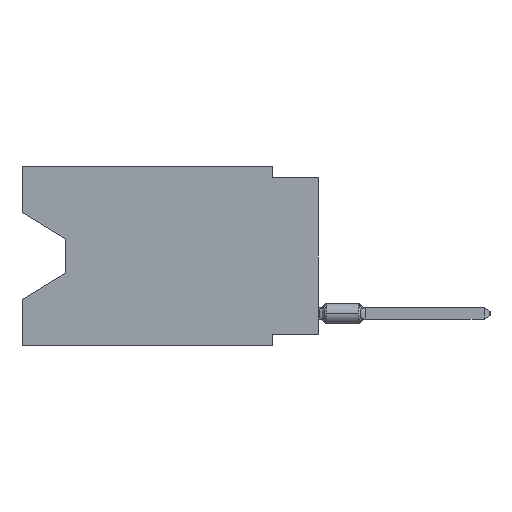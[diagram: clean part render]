
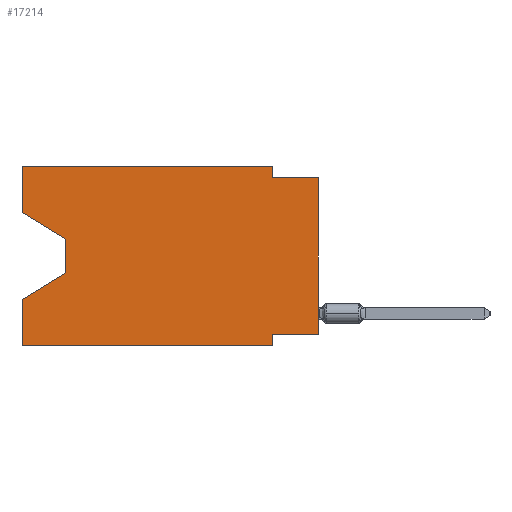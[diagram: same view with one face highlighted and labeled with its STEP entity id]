
A CAD part, left-side view. The second image highlights one B-rep face of the part: STEP entity #17214.
In plain terms, the highlighted planar face has unit normal (-1, 0, 0).
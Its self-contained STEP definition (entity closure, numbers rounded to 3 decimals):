
#974 = LINE ( 'NONE', #6072, #51838 ) ;
#1066 = VERTEX_POINT ( 'NONE', #37199 ) ;
#1993 = DIRECTION ( 'NONE',  ( 0., 0., -1. ) ) ;
#2234 = CARTESIAN_POINT ( 'NONE',  ( 0., 0., -0.635 ) ) ;
#3231 = ORIENTED_EDGE ( 'NONE', *, *, #65630, .T. ) ;
#3848 = CARTESIAN_POINT ( 'NONE',  ( 0., 16.383, -2.546 ) ) ;
#4246 = CARTESIAN_POINT ( 'NONE',  ( 0., 16.383, 0. ) ) ;
#5238 = DIRECTION ( 'NONE',  ( 0., 1., 0. ) ) ;
#5578 = LINE ( 'NONE', #27702, #69295 ) ;
#5609 = DIRECTION ( 'NONE',  ( 0., -0.855, -0.519 ) ) ;
#5758 = CARTESIAN_POINT ( 'NONE',  ( 0., 0., -0.635 ) ) ;
#5978 = EDGE_CURVE ( 'NONE', #13205, #69093, #974, .T. ) ;
#6072 = CARTESIAN_POINT ( 'NONE',  ( 0., 13.97, -5.893 ) ) ;
#9314 = EDGE_CURVE ( 'NONE', #17321, #13205, #5578, .T. ) ;
#12777 = VECTOR ( 'NONE', #44571, 1000. ) ;
#13205 = VERTEX_POINT ( 'NONE', #16826 ) ;
#14056 = VERTEX_POINT ( 'NONE', #45647 ) ;
#14090 = CARTESIAN_POINT ( 'NONE',  ( 0., 16.383, -7.36 ) ) ;
#15935 = PLANE ( 'NONE',  #58836 ) ;
#16826 = CARTESIAN_POINT ( 'NONE',  ( 0., 13.97, -5.893 ) ) ;
#17214 = ADVANCED_FACE ( 'NONE', ( #64526 ), #15935, .F. ) ;
#17321 = VERTEX_POINT ( 'NONE', #65959 ) ;
#18613 = EDGE_CURVE ( 'NONE', #1066, #69093, #59372, .T. ) ;
#20905 = DIRECTION ( 'NONE',  ( 0., 0., 1. ) ) ;
#21351 = DIRECTION ( 'NONE',  ( 0., 0., -1. ) ) ;
#21536 = CARTESIAN_POINT ( 'NONE',  ( 0., 2.54, -9.271 ) ) ;
#23226 = VERTEX_POINT ( 'NONE', #35369 ) ;
#25700 = EDGE_CURVE ( 'NONE', #1066, #67541, #47697, .T. ) ;
#25925 = CARTESIAN_POINT ( 'NONE',  ( 0., 16.383, -9.906 ) ) ;
#26490 = ORIENTED_EDGE ( 'NONE', *, *, #5978, .T. ) ;
#27290 = VECTOR ( 'NONE', #71239, 1000. ) ;
#27702 = CARTESIAN_POINT ( 'NONE',  ( 0., 13.97, -4.013 ) ) ;
#27799 = LINE ( 'NONE', #70962, #63602 ) ;
#28563 = VERTEX_POINT ( 'NONE', #2234 ) ;
#28895 = DIRECTION ( 'NONE',  ( 0., 0.855, -0.519 ) ) ;
#29123 = VECTOR ( 'NONE', #5238, 1000. ) ;
#29581 = VECTOR ( 'NONE', #1993, 1000. ) ;
#30144 = LINE ( 'NONE', #68922, #62560 ) ;
#30364 = DIRECTION ( 'NONE',  ( 0., 0., 1. ) ) ;
#30715 = CARTESIAN_POINT ( 'NONE',  ( 0., 16.383, 0. ) ) ;
#30737 = LINE ( 'NONE', #69533, #29123 ) ;
#31411 = LINE ( 'NONE', #3848, #40615 ) ;
#33691 = ORIENTED_EDGE ( 'NONE', *, *, #54724, .F. ) ;
#33959 = LINE ( 'NONE', #56078, #29581 ) ;
#34143 = ORIENTED_EDGE ( 'NONE', *, *, #60150, .F. ) ;
#35369 = CARTESIAN_POINT ( 'NONE',  ( 0., 2.54, 0. ) ) ;
#35489 = ORIENTED_EDGE ( 'NONE', *, *, #71157, .T. ) ;
#36067 = CARTESIAN_POINT ( 'NONE',  ( 0., 16.383, 0. ) ) ;
#37199 = CARTESIAN_POINT ( 'NONE',  ( 0., 16.383, -9.906 ) ) ;
#37969 = LINE ( 'NONE', #4246, #43032 ) ;
#40615 = VECTOR ( 'NONE', #5609, 1000. ) ;
#41382 = DIRECTION ( 'NONE',  ( 0., -1., 0. ) ) ;
#41470 = VERTEX_POINT ( 'NONE', #43979 ) ;
#42266 = VERTEX_POINT ( 'NONE', #36067 ) ;
#43032 = VECTOR ( 'NONE', #20905, 1000. ) ;
#43979 = CARTESIAN_POINT ( 'NONE',  ( 0., 2.54, -0.635 ) ) ;
#44571 = DIRECTION ( 'NONE',  ( 0., -1., 0. ) ) ;
#44669 = EDGE_CURVE ( 'NONE', #70568, #42266, #37969, .T. ) ;
#45123 = VERTEX_POINT ( 'NONE', #21536 ) ;
#45647 = CARTESIAN_POINT ( 'NONE',  ( 0., 0., -9.271 ) ) ;
#46891 = ORIENTED_EDGE ( 'NONE', *, *, #60630, .F. ) ;
#47697 = LINE ( 'NONE', #25925, #64459 ) ;
#48094 = EDGE_CURVE ( 'NONE', #42266, #23226, #30144, .T. ) ;
#48232 = CARTESIAN_POINT ( 'NONE',  ( 0., 16.383, 0. ) ) ;
#49141 = LINE ( 'NONE', #60372, #27290 ) ;
#49936 = DIRECTION ( 'NONE',  ( 0., 0., -1. ) ) ;
#51178 = CARTESIAN_POINT ( 'NONE',  ( 0., 2.54, -9.906 ) ) ;
#51838 = VECTOR ( 'NONE', #28895, 1000. ) ;
#54724 = EDGE_CURVE ( 'NONE', #45123, #67541, #33959, .T. ) ;
#56078 = CARTESIAN_POINT ( 'NONE',  ( 0., 2.54, -9.906 ) ) ;
#58836 = AXIS2_PLACEMENT_3D ( 'NONE', #48232, #64889, #21351 ) ;
#59372 = LINE ( 'NONE', #30715, #60219 ) ;
#60150 = EDGE_CURVE ( 'NONE', #41470, #28563, #65960, .T. ) ;
#60219 = VECTOR ( 'NONE', #30364, 1000. ) ;
#60372 = CARTESIAN_POINT ( 'NONE',  ( 0., 0., 0. ) ) ;
#60630 = EDGE_CURVE ( 'NONE', #23226, #41470, #27799, .T. ) ;
#61069 = DIRECTION ( 'NONE',  ( 0., 0., -1. ) ) ;
#61179 = ORIENTED_EDGE ( 'NONE', *, *, #48094, .F. ) ;
#61292 = ORIENTED_EDGE ( 'NONE', *, *, #9314, .T. ) ;
#62265 = ORIENTED_EDGE ( 'NONE', *, *, #66811, .F. ) ;
#62560 = VECTOR ( 'NONE', #41382, 1000. ) ;
#62657 = CARTESIAN_POINT ( 'NONE',  ( 0., 16.383, -2.546 ) ) ;
#63602 = VECTOR ( 'NONE', #49936, 1000. ) ;
#64350 = DIRECTION ( 'NONE',  ( 0., -1., 0. ) ) ;
#64459 = VECTOR ( 'NONE', #64350, 1000. ) ;
#64526 = FACE_OUTER_BOUND ( 'NONE', #67720, .T. ) ;
#64889 = DIRECTION ( 'NONE',  ( 1., 0., 0. ) ) ;
#65630 = EDGE_CURVE ( 'NONE', #14056, #28563, #49141, .T. ) ;
#65959 = CARTESIAN_POINT ( 'NONE',  ( 0., 13.97, -4.013 ) ) ;
#65960 = LINE ( 'NONE', #5758, #12777 ) ;
#66501 = ORIENTED_EDGE ( 'NONE', *, *, #44669, .F. ) ;
#66811 = EDGE_CURVE ( 'NONE', #14056, #45123, #30737, .T. ) ;
#67431 = ORIENTED_EDGE ( 'NONE', *, *, #18613, .F. ) ;
#67541 = VERTEX_POINT ( 'NONE', #51178 ) ;
#67720 = EDGE_LOOP ( 'NONE', ( #35489, #61292, #26490, #67431, #68042, #33691, #62265, #3231, #34143, #46891, #61179, #66501 ) ) ;
#68042 = ORIENTED_EDGE ( 'NONE', *, *, #25700, .T. ) ;
#68922 = CARTESIAN_POINT ( 'NONE',  ( 0., 16.383, 0. ) ) ;
#69093 = VERTEX_POINT ( 'NONE', #14090 ) ;
#69295 = VECTOR ( 'NONE', #61069, 1000. ) ;
#69533 = CARTESIAN_POINT ( 'NONE',  ( 0., 0., -9.271 ) ) ;
#70568 = VERTEX_POINT ( 'NONE', #62657 ) ;
#70962 = CARTESIAN_POINT ( 'NONE',  ( 0., 2.54, 0. ) ) ;
#71157 = EDGE_CURVE ( 'NONE', #70568, #17321, #31411, .T. ) ;
#71239 = DIRECTION ( 'NONE',  ( 0., 0., 1. ) ) ;
